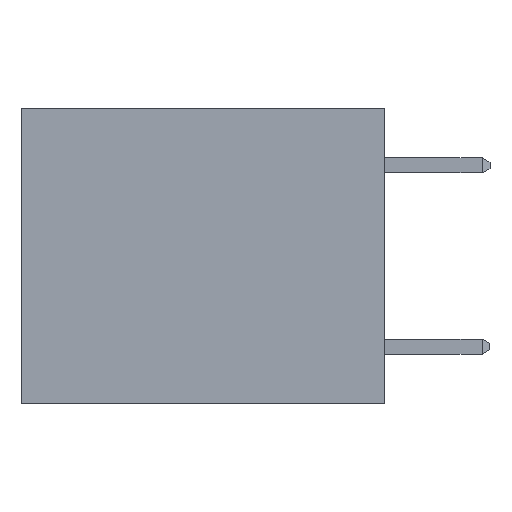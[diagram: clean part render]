
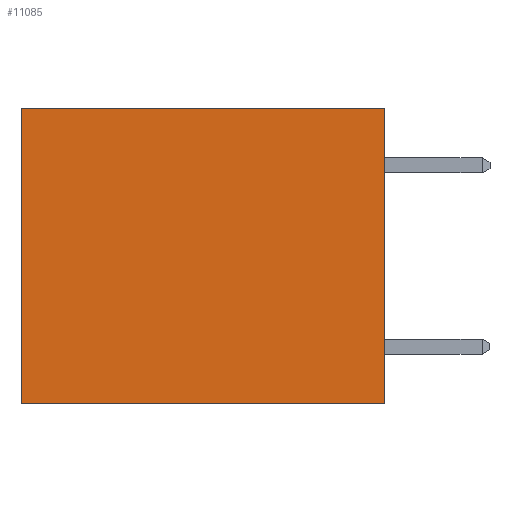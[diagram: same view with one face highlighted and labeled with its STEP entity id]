
A CAD part, left-side view. The second image highlights one B-rep face of the part: STEP entity #11085.
In plain terms, the highlighted planar face has unit normal (-1, 0, 0).
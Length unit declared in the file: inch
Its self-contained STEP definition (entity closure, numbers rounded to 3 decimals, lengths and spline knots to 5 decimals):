
#597 = VERTEX_POINT ( 'NONE', #12364 ) ;
#610 = CARTESIAN_POINT ( 'NONE',  ( 0.3165, 0.6, -0.49 ) ) ;
#1886 = CARTESIAN_POINT ( 'NONE',  ( 0.3165, 0.6, 0. ) ) ;
#2803 = LINE ( 'NONE', #9797, #3967 ) ;
#2882 = PLANE ( 'NONE',  #10090 ) ;
#2995 = CARTESIAN_POINT ( 'NONE',  ( 0.3165, 0.6, -0.49 ) ) ;
#3164 = DIRECTION ( 'NONE',  ( 0., 0., -1. ) ) ;
#3353 = CARTESIAN_POINT ( 'NONE',  ( 0.3165, 0., -0.49 ) ) ;
#3441 = LINE ( 'NONE', #6163, #6018 ) ;
#3713 = DIRECTION ( 'NONE',  ( 0., 1., 0. ) ) ;
#3947 = CARTESIAN_POINT ( 'NONE',  ( 0.3165, 0., -0.49 ) ) ;
#3967 = VECTOR ( 'NONE', #6647, 39.37008 ) ;
#3988 = VERTEX_POINT ( 'NONE', #3353 ) ;
#4937 = DIRECTION ( 'NONE',  ( 0., 0., -1. ) ) ;
#5277 = LINE ( 'NONE', #8851, #6271 ) ;
#6018 = VECTOR ( 'NONE', #3164, 39.37008 ) ;
#6163 = CARTESIAN_POINT ( 'NONE',  ( 0.3165, 0., -0.49 ) ) ;
#6180 = VERTEX_POINT ( 'NONE', #1886 ) ;
#6271 = VECTOR ( 'NONE', #3713, 39.37008 ) ;
#6647 = DIRECTION ( 'NONE',  ( 0., 1., 0. ) ) ;
#7735 = ORIENTED_EDGE ( 'NONE', *, *, #9106, .T. ) ;
#7776 = DIRECTION ( 'NONE',  ( 0., 0., -1. ) ) ;
#8481 = EDGE_LOOP ( 'NONE', ( #7735, #8901, #10411, #11370 ) ) ;
#8851 = CARTESIAN_POINT ( 'NONE',  ( 0.3165, 0., -0.49 ) ) ;
#8901 = ORIENTED_EDGE ( 'NONE', *, *, #12600, .F. ) ;
#9106 = EDGE_CURVE ( 'NONE', #6180, #9881, #9398, .T. ) ;
#9398 = LINE ( 'NONE', #610, #12667 ) ;
#9797 = CARTESIAN_POINT ( 'NONE',  ( 0.3165, 0., 0. ) ) ;
#9881 = VERTEX_POINT ( 'NONE', #2995 ) ;
#10090 = AXIS2_PLACEMENT_3D ( 'NONE', #3947, #11270, #4937 ) ;
#10411 = ORIENTED_EDGE ( 'NONE', *, *, #11225, .F. ) ;
#10712 = FACE_OUTER_BOUND ( 'NONE', #8481, .T. ) ;
#11085 = ADVANCED_FACE ( 'NONE', ( #10712 ), #2882, .F. ) ;
#11225 = EDGE_CURVE ( 'NONE', #597, #3988, #3441, .T. ) ;
#11270 = DIRECTION ( 'NONE',  ( 1., 0., 0. ) ) ;
#11370 = ORIENTED_EDGE ( 'NONE', *, *, #12305, .T. ) ;
#12305 = EDGE_CURVE ( 'NONE', #597, #6180, #2803, .T. ) ;
#12364 = CARTESIAN_POINT ( 'NONE',  ( 0.3165, 0., 0. ) ) ;
#12600 = EDGE_CURVE ( 'NONE', #3988, #9881, #5277, .T. ) ;
#12667 = VECTOR ( 'NONE', #7776, 39.37008 ) ;
